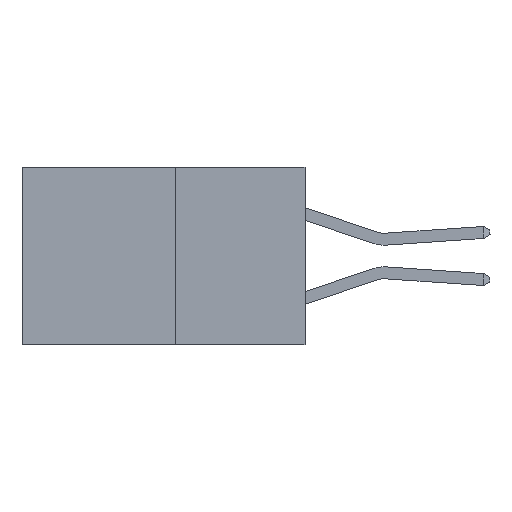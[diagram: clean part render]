
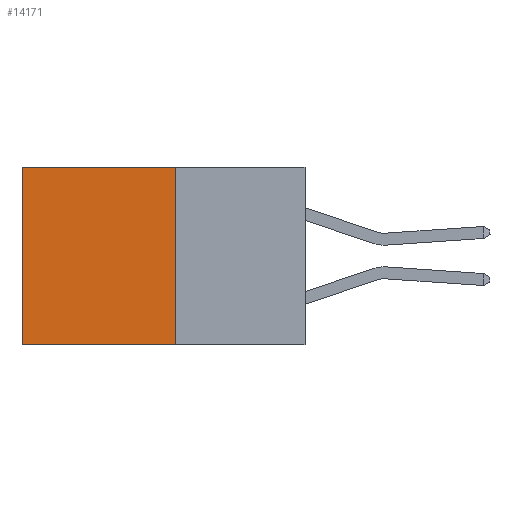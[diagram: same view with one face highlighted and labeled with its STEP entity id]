
A CAD part, left-side view. The second image highlights one B-rep face of the part: STEP entity #14171.
In plain terms, the highlighted planar face has unit normal (-1, 0, 0).
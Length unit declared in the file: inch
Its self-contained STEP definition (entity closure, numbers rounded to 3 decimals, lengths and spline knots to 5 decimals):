
#174 = EDGE_CURVE ( 'NONE', #7504, #11915, #5294, .T. ) ;
#233 = VERTEX_POINT ( 'NONE', #4477 ) ;
#476 = DIRECTION ( 'NONE',  ( 0., 1., 0. ) ) ;
#616 = EDGE_CURVE ( 'NONE', #6967, #233, #10629, .T. ) ;
#928 = VECTOR ( 'NONE', #476, 39.37008 ) ;
#1023 = FACE_OUTER_BOUND ( 'NONE', #4990, .T. ) ;
#1262 = VECTOR ( 'NONE', #10777, 39.37008 ) ;
#1388 = CARTESIAN_POINT ( 'NONE',  ( 0.277, 0.27, -0.37 ) ) ;
#1761 = DIRECTION ( 'NONE',  ( 0., 1., 0. ) ) ;
#1788 = LINE ( 'NONE', #18794, #1262 ) ;
#2289 = ORIENTED_EDGE ( 'NONE', *, *, #13802, .F. ) ;
#4477 = CARTESIAN_POINT ( 'NONE',  ( 0.277, 0.59, 0. ) ) ;
#4829 = CARTESIAN_POINT ( 'NONE',  ( 0.277, 0.27, 0. ) ) ;
#4990 = EDGE_LOOP ( 'NONE', ( #12811, #14110, #2289, #11343 ) ) ;
#5294 = LINE ( 'NONE', #7417, #928 ) ;
#5819 = CARTESIAN_POINT ( 'NONE',  ( 0.277, 0.27, -0.37 ) ) ;
#6967 = VERTEX_POINT ( 'NONE', #9380 ) ;
#7417 = CARTESIAN_POINT ( 'NONE',  ( 0.277, 0.27, -0.37 ) ) ;
#7504 = VERTEX_POINT ( 'NONE', #9087 ) ;
#8246 = VECTOR ( 'NONE', #9556, 39.37008 ) ;
#9087 = CARTESIAN_POINT ( 'NONE',  ( 0.277, 0.27, -0.37 ) ) ;
#9123 = DIRECTION ( 'NONE',  ( 1., 0., 0. ) ) ;
#9380 = CARTESIAN_POINT ( 'NONE',  ( 0.277, 0.27, 0. ) ) ;
#9556 = DIRECTION ( 'NONE',  ( 0., 0., -1. ) ) ;
#10132 = VECTOR ( 'NONE', #1761, 39.37008 ) ;
#10629 = LINE ( 'NONE', #4829, #10132 ) ;
#10777 = DIRECTION ( 'NONE',  ( 0., 0., -1. ) ) ;
#11343 = ORIENTED_EDGE ( 'NONE', *, *, #616, .T. ) ;
#11915 = VERTEX_POINT ( 'NONE', #19034 ) ;
#12811 = ORIENTED_EDGE ( 'NONE', *, *, #14882, .T. ) ;
#13802 = EDGE_CURVE ( 'NONE', #6967, #7504, #16825, .T. ) ;
#14110 = ORIENTED_EDGE ( 'NONE', *, *, #174, .F. ) ;
#14171 = ADVANCED_FACE ( 'NONE', ( #1023 ), #15530, .F. ) ;
#14882 = EDGE_CURVE ( 'NONE', #233, #11915, #1788, .T. ) ;
#15530 = PLANE ( 'NONE',  #18121 ) ;
#16825 = LINE ( 'NONE', #1388, #8246 ) ;
#18121 = AXIS2_PLACEMENT_3D ( 'NONE', #5819, #9123, #20329 ) ;
#18794 = CARTESIAN_POINT ( 'NONE',  ( 0.277, 0.59, -0.37 ) ) ;
#19034 = CARTESIAN_POINT ( 'NONE',  ( 0.277, 0.59, -0.37 ) ) ;
#20329 = DIRECTION ( 'NONE',  ( 0., 0., -1. ) ) ;
